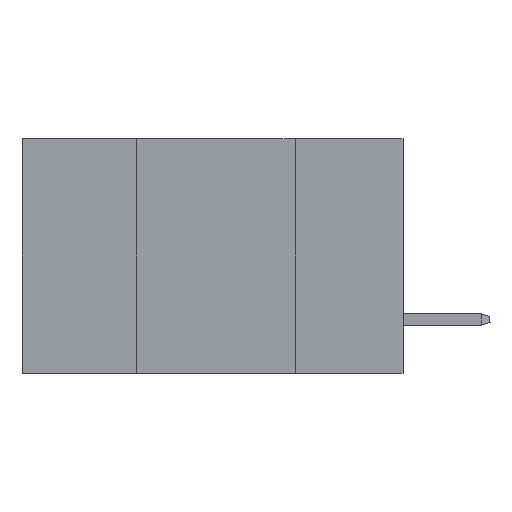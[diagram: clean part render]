
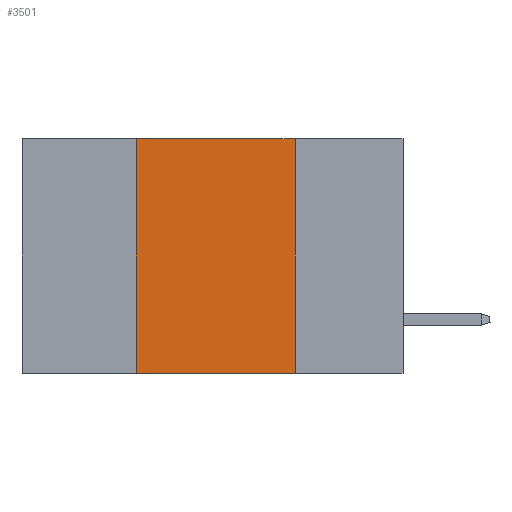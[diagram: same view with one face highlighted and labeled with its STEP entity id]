
A CAD part, left-side view. The second image highlights one B-rep face of the part: STEP entity #3501.
In plain terms, the highlighted planar face has unit normal (-1, 0, 0).
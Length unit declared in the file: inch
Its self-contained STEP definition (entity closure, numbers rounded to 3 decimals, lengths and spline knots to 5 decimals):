
#771 = ORIENTED_EDGE ( 'NONE', *, *, #9132, .F. ) ;
#1301 = LINE ( 'NONE', #11665, #3025 ) ;
#1687 = PLANE ( 'NONE',  #11313 ) ;
#1975 = VERTEX_POINT ( 'NONE', #19946 ) ;
#2168 = LINE ( 'NONE', #7347, #18631 ) ;
#2490 = VERTEX_POINT ( 'NONE', #17295 ) ;
#2647 = VERTEX_POINT ( 'NONE', #9972 ) ;
#2953 = DIRECTION ( 'NONE',  ( 1., 0., 0. ) ) ;
#3025 = VECTOR ( 'NONE', #15292, 39.37008 ) ;
#3501 = ADVANCED_FACE ( 'NONE', ( #11945 ), #1687, .F. ) ;
#6157 = CARTESIAN_POINT ( 'NONE',  ( 0., 0.42, -0.37 ) ) ;
#6617 = LINE ( 'NONE', #20649, #20651 ) ;
#6949 = CARTESIAN_POINT ( 'NONE',  ( 0., 0.6, 0. ) ) ;
#7056 = EDGE_CURVE ( 'NONE', #20783, #2647, #6617, .T. ) ;
#7347 = CARTESIAN_POINT ( 'NONE',  ( 0., 0.17, 0. ) ) ;
#9132 = EDGE_CURVE ( 'NONE', #2490, #2647, #2168, .T. ) ;
#9151 = DIRECTION ( 'NONE',  ( 0., 0., -1. ) ) ;
#9972 = CARTESIAN_POINT ( 'NONE',  ( 0., 0.17, -0.37 ) ) ;
#10711 = EDGE_CURVE ( 'NONE', #20783, #1975, #1301, .T. ) ;
#11313 = AXIS2_PLACEMENT_3D ( 'NONE', #20315, #2953, #19281 ) ;
#11665 = CARTESIAN_POINT ( 'NONE',  ( 0., 0.42, 0. ) ) ;
#11945 = FACE_OUTER_BOUND ( 'NONE', #16801, .T. ) ;
#12045 = DIRECTION ( 'NONE',  ( 0., -1., 0. ) ) ;
#13951 = ORIENTED_EDGE ( 'NONE', *, *, #7056, .T. ) ;
#15292 = DIRECTION ( 'NONE',  ( 0., 0., 1. ) ) ;
#16801 = EDGE_LOOP ( 'NONE', ( #771, #18421, #20801, #13951 ) ) ;
#16857 = DIRECTION ( 'NONE',  ( 0., -1., 0. ) ) ;
#17295 = CARTESIAN_POINT ( 'NONE',  ( 0., 0.17, 0. ) ) ;
#18421 = ORIENTED_EDGE ( 'NONE', *, *, #21784, .F. ) ;
#18631 = VECTOR ( 'NONE', #9151, 39.37008 ) ;
#19281 = DIRECTION ( 'NONE',  ( 0., 0., -1. ) ) ;
#19455 = VECTOR ( 'NONE', #16857, 39.37008 ) ;
#19946 = CARTESIAN_POINT ( 'NONE',  ( 0., 0.42, 0. ) ) ;
#20315 = CARTESIAN_POINT ( 'NONE',  ( 0., 0.6, 0. ) ) ;
#20649 = CARTESIAN_POINT ( 'NONE',  ( 0., 0.6, -0.37 ) ) ;
#20651 = VECTOR ( 'NONE', #12045, 39.37008 ) ;
#20767 = LINE ( 'NONE', #6949, #19455 ) ;
#20783 = VERTEX_POINT ( 'NONE', #6157 ) ;
#20801 = ORIENTED_EDGE ( 'NONE', *, *, #10711, .F. ) ;
#21784 = EDGE_CURVE ( 'NONE', #1975, #2490, #20767, .T. ) ;
